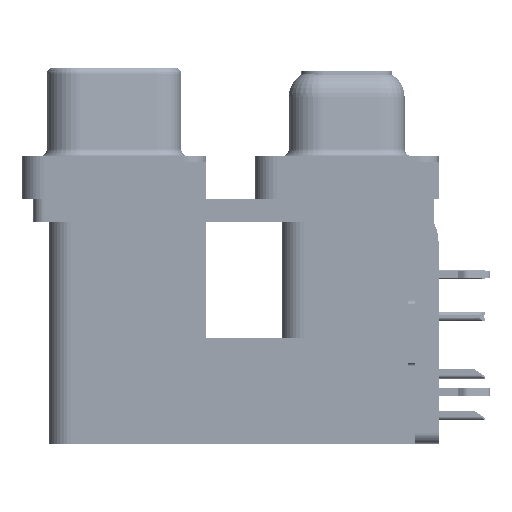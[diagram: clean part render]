
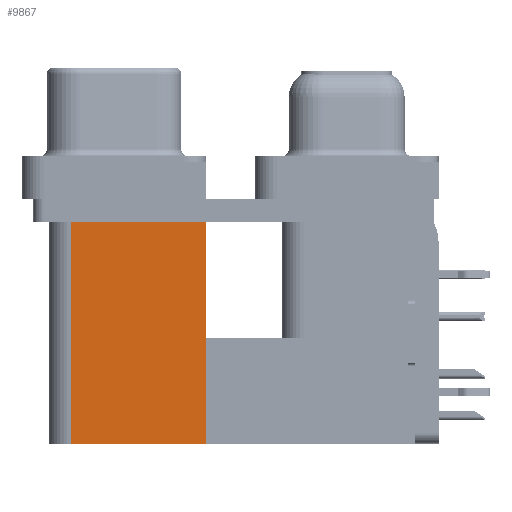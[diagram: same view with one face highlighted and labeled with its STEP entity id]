
A CAD part, left-side view. The second image highlights one B-rep face of the part: STEP entity #9867.
In plain terms, the highlighted planar face has unit normal (-1, 0, 0).
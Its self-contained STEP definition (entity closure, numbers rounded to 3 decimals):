
#728 = DIRECTION ( 'NONE',  ( 1., 0., 0. ) ) ;
#4481 = CARTESIAN_POINT ( 'NONE',  ( 3.79, 18.8, -2.5 ) ) ;
#4962 = CARTESIAN_POINT ( 'NONE',  ( 3.79, 9.6, -19.2 ) ) ;
#5205 = ORIENTED_EDGE ( 'NONE', *, *, #37178, .T. ) ;
#9751 = DIRECTION ( 'NONE',  ( 0., 0., 1. ) ) ;
#9867 = ADVANCED_FACE ( 'NONE', ( #33766 ), #16713, .F. ) ;
#10249 = CARTESIAN_POINT ( 'NONE',  ( 3.79, 9.6, -2.5 ) ) ;
#12043 = LINE ( 'NONE', #55810, #51028 ) ;
#15095 = LINE ( 'NONE', #58869, #21448 ) ;
#16648 = EDGE_CURVE ( 'NONE', #31855, #20061, #42974, .T. ) ;
#16713 = PLANE ( 'NONE',  #62176 ) ;
#20061 = VERTEX_POINT ( 'NONE', #58090 ) ;
#21448 = VECTOR ( 'NONE', #9751, 1000. ) ;
#22027 = CARTESIAN_POINT ( 'NONE',  ( 3.79, 9.6, -19.2 ) ) ;
#25940 = VERTEX_POINT ( 'NONE', #4481 ) ;
#29788 = VERTEX_POINT ( 'NONE', #40473 ) ;
#31570 = DIRECTION ( 'NONE',  ( 0., 1., 0. ) ) ;
#31592 = EDGE_CURVE ( 'NONE', #29788, #25940, #15095, .T. ) ;
#31855 = VERTEX_POINT ( 'NONE', #4962 ) ;
#31970 = EDGE_CURVE ( 'NONE', #31855, #29788, #12043, .T. ) ;
#33766 = FACE_OUTER_BOUND ( 'NONE', #41176, .T. ) ;
#36234 = ORIENTED_EDGE ( 'NONE', *, *, #31592, .F. ) ;
#37178 = EDGE_CURVE ( 'NONE', #20061, #25940, #54358, .T. ) ;
#40427 = ORIENTED_EDGE ( 'NONE', *, *, #16648, .T. ) ;
#40473 = CARTESIAN_POINT ( 'NONE',  ( 3.79, 18.8, -19.2 ) ) ;
#41176 = EDGE_LOOP ( 'NONE', ( #5205, #36234, #47979, #40427 ) ) ;
#42974 = LINE ( 'NONE', #65373, #65223 ) ;
#47979 = ORIENTED_EDGE ( 'NONE', *, *, #31970, .F. ) ;
#51028 = VECTOR ( 'NONE', #56511, 1000. ) ;
#54018 = DIRECTION ( 'NONE',  ( 0., 0., 1. ) ) ;
#54358 = LINE ( 'NONE', #10249, #55805 ) ;
#55805 = VECTOR ( 'NONE', #31570, 1000. ) ;
#55810 = CARTESIAN_POINT ( 'NONE',  ( 3.79, 9.6, -19.2 ) ) ;
#56511 = DIRECTION ( 'NONE',  ( 0., 1., 0. ) ) ;
#58090 = CARTESIAN_POINT ( 'NONE',  ( 3.79, 9.6, -2.5 ) ) ;
#58869 = CARTESIAN_POINT ( 'NONE',  ( 3.79, 18.8, -19.2 ) ) ;
#59786 = DIRECTION ( 'NONE',  ( 0., 0., -1. ) ) ;
#62176 = AXIS2_PLACEMENT_3D ( 'NONE', #22027, #728, #59786 ) ;
#65223 = VECTOR ( 'NONE', #54018, 1000. ) ;
#65373 = CARTESIAN_POINT ( 'NONE',  ( 3.79, 9.6, -19.2 ) ) ;
